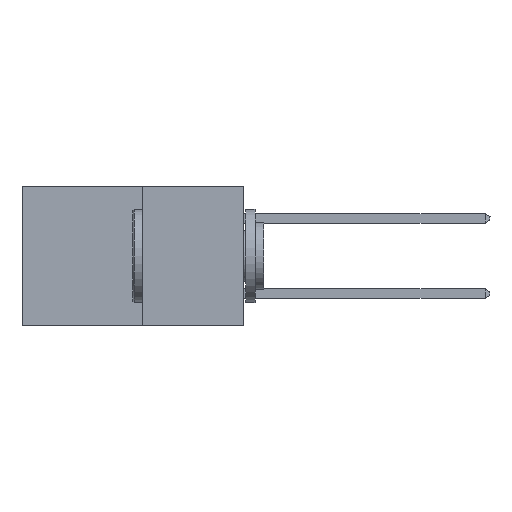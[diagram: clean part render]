
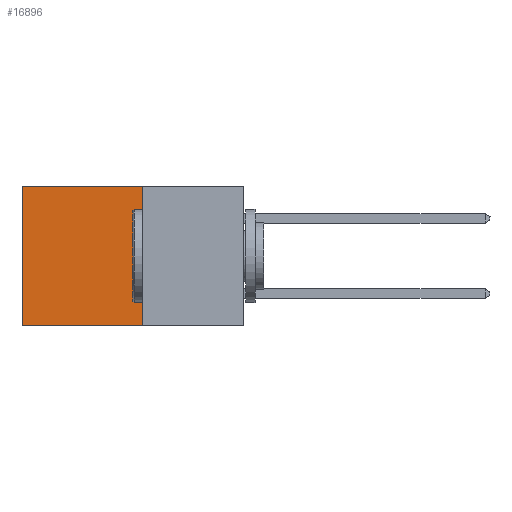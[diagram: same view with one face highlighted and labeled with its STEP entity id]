
A CAD part, left-side view. The second image highlights one B-rep face of the part: STEP entity #16896.
In plain terms, the highlighted planar face has unit normal (-1, 0, 0).
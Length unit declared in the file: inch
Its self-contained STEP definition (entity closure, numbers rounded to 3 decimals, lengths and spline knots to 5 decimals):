
#253 = VECTOR ( 'NONE', #21466, 39.37008 ) ;
#281 = CARTESIAN_POINT ( 'NONE',  ( 0.277, 0.59, -0.37 ) ) ;
#373 = LINE ( 'NONE', #22155, #19334 ) ;
#1437 = EDGE_CURVE ( 'NONE', #5421, #10284, #5467, .T. ) ;
#2033 = VECTOR ( 'NONE', #24925, 39.37008 ) ;
#2597 = FACE_OUTER_BOUND ( 'NONE', #6792, .T. ) ;
#2784 = DIRECTION ( 'NONE',  ( 0., 0., -1. ) ) ;
#2792 = ORIENTED_EDGE ( 'NONE', *, *, #24749, .T. ) ;
#4591 = CARTESIAN_POINT ( 'NONE',  ( 0.277, 0.27, -0.37 ) ) ;
#4703 = CARTESIAN_POINT ( 'NONE',  ( 0.277, 0.27, -0.37 ) ) ;
#5139 = ORIENTED_EDGE ( 'NONE', *, *, #15877, .T. ) ;
#5421 = VERTEX_POINT ( 'NONE', #14291 ) ;
#5467 = LINE ( 'NONE', #22794, #253 ) ;
#5743 = CARTESIAN_POINT ( 'NONE',  ( 0.277, 0.59, -0.37 ) ) ;
#5834 = CARTESIAN_POINT ( 'NONE',  ( 0.277, 0.59, 0. ) ) ;
#6217 = VERTEX_POINT ( 'NONE', #5834 ) ;
#6792 = EDGE_LOOP ( 'NONE', ( #5139, #7648, #19560, #2792 ) ) ;
#7648 = ORIENTED_EDGE ( 'NONE', *, *, #24858, .F. ) ;
#10284 = VERTEX_POINT ( 'NONE', #4591 ) ;
#14291 = CARTESIAN_POINT ( 'NONE',  ( 0.277, 0.27, 0. ) ) ;
#14612 = DIRECTION ( 'NONE',  ( 1., 0., 0. ) ) ;
#15188 = AXIS2_PLACEMENT_3D ( 'NONE', #4703, #14612, #2784 ) ;
#15877 = EDGE_CURVE ( 'NONE', #6217, #17362, #17687, .T. ) ;
#16550 = DIRECTION ( 'NONE',  ( 0., 1., 0. ) ) ;
#16789 = CARTESIAN_POINT ( 'NONE',  ( 0.277, 0.27, -0.37 ) ) ;
#16896 = ADVANCED_FACE ( 'NONE', ( #2597 ), #24014, .F. ) ;
#16945 = VECTOR ( 'NONE', #20601, 39.37008 ) ;
#17362 = VERTEX_POINT ( 'NONE', #281 ) ;
#17687 = LINE ( 'NONE', #5743, #2033 ) ;
#19334 = VECTOR ( 'NONE', #16550, 39.37008 ) ;
#19560 = ORIENTED_EDGE ( 'NONE', *, *, #1437, .F. ) ;
#20601 = DIRECTION ( 'NONE',  ( 0., 1., 0. ) ) ;
#21466 = DIRECTION ( 'NONE',  ( 0., 0., -1. ) ) ;
#22155 = CARTESIAN_POINT ( 'NONE',  ( 0.277, 0.27, 0. ) ) ;
#22794 = CARTESIAN_POINT ( 'NONE',  ( 0.277, 0.27, -0.37 ) ) ;
#23151 = LINE ( 'NONE', #16789, #16945 ) ;
#24014 = PLANE ( 'NONE',  #15188 ) ;
#24749 = EDGE_CURVE ( 'NONE', #5421, #6217, #373, .T. ) ;
#24858 = EDGE_CURVE ( 'NONE', #10284, #17362, #23151, .T. ) ;
#24925 = DIRECTION ( 'NONE',  ( 0., 0., -1. ) ) ;
